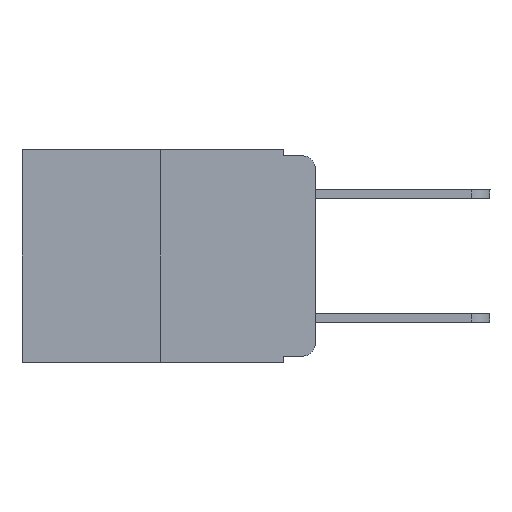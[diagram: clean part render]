
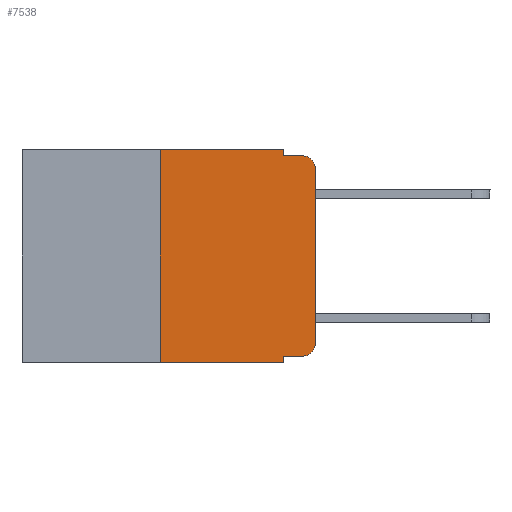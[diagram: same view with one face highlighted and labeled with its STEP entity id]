
A CAD part, left-side view. The second image highlights one B-rep face of the part: STEP entity #7538.
In plain terms, the highlighted planar face has unit normal (-1, 0, 0).
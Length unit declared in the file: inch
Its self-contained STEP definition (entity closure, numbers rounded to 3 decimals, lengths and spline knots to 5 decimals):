
#139 = CARTESIAN_POINT ( 'NONE',  ( 0., 0., -0.03 ) ) ;
#187 = VERTEX_POINT ( 'NONE', #218 ) ;
#218 = CARTESIAN_POINT ( 'NONE',  ( 0., 0.051, -0.01 ) ) ;
#251 = DIRECTION ( 'NONE',  ( 1., 0., 0. ) ) ;
#275 = CIRCLE ( 'NONE', #3075, 0.02 ) ;
#279 = LINE ( 'NONE', #3547, #8008 ) ;
#547 = LINE ( 'NONE', #8635, #12941 ) ;
#566 = CARTESIAN_POINT ( 'NONE',  ( 0., 0.473, -0.343 ) ) ;
#659 = ORIENTED_EDGE ( 'NONE', *, *, #3138, .F. ) ;
#956 = CARTESIAN_POINT ( 'NONE',  ( 0., 0., 0. ) ) ;
#1105 = ORIENTED_EDGE ( 'NONE', *, *, #2693, .F. ) ;
#1140 = DIRECTION ( 'NONE',  ( 0., 0., -1. ) ) ;
#1193 = ORIENTED_EDGE ( 'NONE', *, *, #7565, .T. ) ;
#1352 = DIRECTION ( 'NONE',  ( 0., -1., 0. ) ) ;
#1756 = CARTESIAN_POINT ( 'NONE',  ( 0., 0.051, -0.343 ) ) ;
#2100 = DIRECTION ( 'NONE',  ( 0., 0., 1. ) ) ;
#2149 = DIRECTION ( 'NONE',  ( -1., 0., 0. ) ) ;
#2404 = CARTESIAN_POINT ( 'NONE',  ( 0., 0.473, 0. ) ) ;
#2466 = VECTOR ( 'NONE', #11210, 39.37008 ) ;
#2570 = EDGE_CURVE ( 'NONE', #4333, #187, #2712, .T. ) ;
#2693 = EDGE_CURVE ( 'NONE', #8964, #8783, #12218, .T. ) ;
#2712 = LINE ( 'NONE', #8925, #6290 ) ;
#2807 = EDGE_CURVE ( 'NONE', #13111, #4333, #547, .T. ) ;
#2811 = AXIS2_PLACEMENT_3D ( 'NONE', #2404, #251, #11383 ) ;
#3075 = AXIS2_PLACEMENT_3D ( 'NONE', #4886, #2149, #1140 ) ;
#3138 = EDGE_CURVE ( 'NONE', #187, #11513, #4017, .T. ) ;
#3166 = VERTEX_POINT ( 'NONE', #139 ) ;
#3276 = DIRECTION ( 'NONE',  ( -1., 0., 0. ) ) ;
#3339 = FACE_OUTER_BOUND ( 'NONE', #7810, .T. ) ;
#3547 = CARTESIAN_POINT ( 'NONE',  ( 0., 0.25, 0. ) ) ;
#4017 = LINE ( 'NONE', #6014, #8245 ) ;
#4219 = CARTESIAN_POINT ( 'NONE',  ( 0., 0.051, 0. ) ) ;
#4333 = VERTEX_POINT ( 'NONE', #4219 ) ;
#4352 = DIRECTION ( 'NONE',  ( 0., 0., 1. ) ) ;
#4418 = EDGE_CURVE ( 'NONE', #5989, #3166, #7295, .T. ) ;
#4556 = LINE ( 'NONE', #566, #12291 ) ;
#4765 = VERTEX_POINT ( 'NONE', #8085 ) ;
#4886 = CARTESIAN_POINT ( 'NONE',  ( 0., 0.02, -0.03 ) ) ;
#5271 = CARTESIAN_POINT ( 'NONE',  ( 0., 0.02, -0.313 ) ) ;
#5930 = ORIENTED_EDGE ( 'NONE', *, *, #8155, .T. ) ;
#5989 = VERTEX_POINT ( 'NONE', #6746 ) ;
#6014 = CARTESIAN_POINT ( 'NONE',  ( 0., 0.051, -0.01 ) ) ;
#6290 = VECTOR ( 'NONE', #7910, 39.37008 ) ;
#6419 = CIRCLE ( 'NONE', #12004, 0.02 ) ;
#6647 = LINE ( 'NONE', #9813, #11103 ) ;
#6746 = CARTESIAN_POINT ( 'NONE',  ( 0., 0., -0.313 ) ) ;
#6852 = DIRECTION ( 'NONE',  ( 0., -1., 0. ) ) ;
#7295 = LINE ( 'NONE', #956, #11629 ) ;
#7429 = ORIENTED_EDGE ( 'NONE', *, *, #2807, .F. ) ;
#7439 = VERTEX_POINT ( 'NONE', #11182 ) ;
#7461 = ORIENTED_EDGE ( 'NONE', *, *, #8808, .T. ) ;
#7538 = ADVANCED_FACE ( 'NONE', ( #3339 ), #12451, .F. ) ;
#7565 = EDGE_CURVE ( 'NONE', #4765, #5989, #6419, .T. ) ;
#7697 = ORIENTED_EDGE ( 'NONE', *, *, #2570, .F. ) ;
#7810 = EDGE_LOOP ( 'NONE', ( #12216, #7461, #659, #7697, #7429, #11541, #11644, #1105, #5930, #1193 ) ) ;
#7910 = DIRECTION ( 'NONE',  ( 0., 0., -1. ) ) ;
#8008 = VECTOR ( 'NONE', #4352, 39.37008 ) ;
#8085 = CARTESIAN_POINT ( 'NONE',  ( 0., 0.02, -0.333 ) ) ;
#8155 = EDGE_CURVE ( 'NONE', #8964, #4765, #6647, .T. ) ;
#8238 = DIRECTION ( 'NONE',  ( 0., -1., 0. ) ) ;
#8245 = VECTOR ( 'NONE', #8238, 39.37008 ) ;
#8635 = CARTESIAN_POINT ( 'NONE',  ( 0., 0.473, 0. ) ) ;
#8783 = VERTEX_POINT ( 'NONE', #1756 ) ;
#8808 = EDGE_CURVE ( 'NONE', #3166, #11513, #275, .T. ) ;
#8925 = CARTESIAN_POINT ( 'NONE',  ( 0., 0.051, 0. ) ) ;
#8964 = VERTEX_POINT ( 'NONE', #10569 ) ;
#9813 = CARTESIAN_POINT ( 'NONE',  ( 0., 0.051, -0.333 ) ) ;
#10450 = DIRECTION ( 'NONE',  ( 0., 0., -1. ) ) ;
#10569 = CARTESIAN_POINT ( 'NONE',  ( 0., 0.051, -0.333 ) ) ;
#11015 = CARTESIAN_POINT ( 'NONE',  ( 0., 0.25, 0. ) ) ;
#11103 = VECTOR ( 'NONE', #6852, 39.37008 ) ;
#11182 = CARTESIAN_POINT ( 'NONE',  ( 0., 0.25, -0.343 ) ) ;
#11210 = DIRECTION ( 'NONE',  ( 0., 0., -1. ) ) ;
#11383 = DIRECTION ( 'NONE',  ( 0., 0., -1. ) ) ;
#11403 = CARTESIAN_POINT ( 'NONE',  ( 0., 0.051, 0. ) ) ;
#11513 = VERTEX_POINT ( 'NONE', #12365 ) ;
#11541 = ORIENTED_EDGE ( 'NONE', *, *, #12082, .F. ) ;
#11629 = VECTOR ( 'NONE', #2100, 39.37008 ) ;
#11644 = ORIENTED_EDGE ( 'NONE', *, *, #11657, .T. ) ;
#11657 = EDGE_CURVE ( 'NONE', #7439, #8783, #4556, .T. ) ;
#12004 = AXIS2_PLACEMENT_3D ( 'NONE', #5271, #3276, #10450 ) ;
#12082 = EDGE_CURVE ( 'NONE', #7439, #13111, #279, .T. ) ;
#12216 = ORIENTED_EDGE ( 'NONE', *, *, #4418, .T. ) ;
#12218 = LINE ( 'NONE', #11403, #2466 ) ;
#12291 = VECTOR ( 'NONE', #12688, 39.37008 ) ;
#12365 = CARTESIAN_POINT ( 'NONE',  ( 0., 0.02, -0.01 ) ) ;
#12451 = PLANE ( 'NONE',  #2811 ) ;
#12688 = DIRECTION ( 'NONE',  ( 0., -1., 0. ) ) ;
#12941 = VECTOR ( 'NONE', #1352, 39.37008 ) ;
#13111 = VERTEX_POINT ( 'NONE', #11015 ) ;
